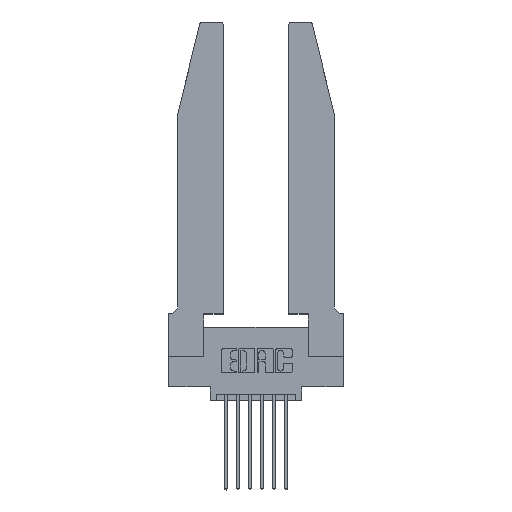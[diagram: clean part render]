
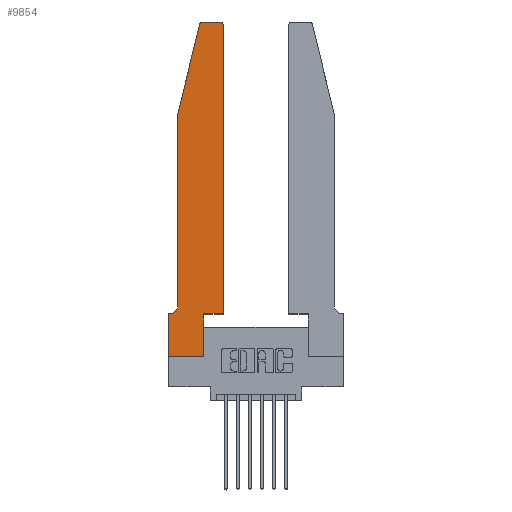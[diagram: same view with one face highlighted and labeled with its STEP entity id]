
A CAD part, top view. The second image highlights one B-rep face of the part: STEP entity #9854.
In plain terms, the highlighted planar face has unit normal (0, 0, 1).
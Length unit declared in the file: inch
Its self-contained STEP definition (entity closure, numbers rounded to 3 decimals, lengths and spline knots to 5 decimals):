
#182 = VECTOR ( 'NONE', #11333, 39.37008 ) ;
#217 = DIRECTION ( 'NONE',  ( 0., 0., 1. ) ) ;
#329 = EDGE_CURVE ( 'NONE', #9574, #2179, #9355, .T. ) ;
#673 = VECTOR ( 'NONE', #8299, 39.37008 ) ;
#785 = ORIENTED_EDGE ( 'NONE', *, *, #9472, .T. ) ;
#1002 = LINE ( 'NONE', #8982, #1178 ) ;
#1145 = EDGE_CURVE ( 'NONE', #2179, #4719, #1292, .T. ) ;
#1178 = VECTOR ( 'NONE', #5602, 39.37008 ) ;
#1292 = LINE ( 'NONE', #14469, #14394 ) ;
#1316 = DIRECTION ( 'NONE',  ( 1., 0., 0. ) ) ;
#1964 = ORIENTED_EDGE ( 'NONE', *, *, #12261, .T. ) ;
#2009 = CARTESIAN_POINT ( 'NONE',  ( 0.25487, 2.72718, 0.37 ) ) ;
#2179 = VERTEX_POINT ( 'NONE', #2859 ) ;
#2706 = CARTESIAN_POINT ( 'NONE',  ( 0.2865, 0., 0.37 ) ) ;
#2859 = CARTESIAN_POINT ( 'NONE',  ( 0.0055, 0.35, 0.37 ) ) ;
#3103 = LINE ( 'NONE', #12303, #9683 ) ;
#3214 = CARTESIAN_POINT ( 'NONE',  ( 0.2865, 0.35, 0.37 ) ) ;
#3313 = PLANE ( 'NONE',  #5761 ) ;
#3316 = VERTEX_POINT ( 'NONE', #2706 ) ;
#3802 = CIRCLE ( 'NONE', #13744, 0.03 ) ;
#3925 = CARTESIAN_POINT ( 'NONE',  ( 0.4505, 0.35, 0.37 ) ) ;
#3987 = LINE ( 'NONE', #7133, #673 ) ;
#4119 = CARTESIAN_POINT ( 'NONE',  ( 0., 0., 0.37 ) ) ;
#4132 = FACE_OUTER_BOUND ( 'NONE', #8071, .T. ) ;
#4164 = VECTOR ( 'NONE', #7392, 39.37008 ) ;
#4212 = VERTEX_POINT ( 'NONE', #10690 ) ;
#4330 = ORIENTED_EDGE ( 'NONE', *, *, #10019, .T. ) ;
#4646 = VECTOR ( 'NONE', #11524, 39.37008 ) ;
#4649 = DIRECTION ( 'NONE',  ( -0.239, -0.971, 0. ) ) ;
#4719 = VERTEX_POINT ( 'NONE', #6005 ) ;
#4817 = VERTEX_POINT ( 'NONE', #4119 ) ;
#4819 = LINE ( 'NONE', #10349, #6881 ) ;
#5023 = EDGE_CURVE ( 'NONE', #11621, #13832, #3103, .T. ) ;
#5448 = EDGE_CURVE ( 'NONE', #3316, #9786, #7367, .T. ) ;
#5484 = CARTESIAN_POINT ( 'NONE',  ( 0.0755, 0.42, 0.37 ) ) ;
#5602 = DIRECTION ( 'NONE',  ( -1., 0., 0. ) ) ;
#5709 = DIRECTION ( 'NONE',  ( 0., 0., -1. ) ) ;
#5761 = AXIS2_PLACEMENT_3D ( 'NONE', #13347, #9991, #11146 ) ;
#5821 = ORIENTED_EDGE ( 'NONE', *, *, #11363, .T. ) ;
#6005 = CARTESIAN_POINT ( 'NONE',  ( 0., 0.35, 0.37 ) ) ;
#6082 = ORIENTED_EDGE ( 'NONE', *, *, #7793, .T. ) ;
#6100 = ORIENTED_EDGE ( 'NONE', *, *, #5448, .T. ) ;
#6203 = ORIENTED_EDGE ( 'NONE', *, *, #1145, .T. ) ;
#6380 = AXIS2_PLACEMENT_3D ( 'NONE', #10521, #10358, #11460 ) ;
#6488 = CARTESIAN_POINT ( 'NONE',  ( 0., 0., 0.37 ) ) ;
#6531 = VECTOR ( 'NONE', #1316, 39.37008 ) ;
#6545 = VERTEX_POINT ( 'NONE', #3925 ) ;
#6563 = DIRECTION ( 'NONE',  ( -1., 0., 0. ) ) ;
#6828 = CARTESIAN_POINT ( 'NONE',  ( 0.4505, 0.35, 0.37 ) ) ;
#6881 = VECTOR ( 'NONE', #9256, 39.37008 ) ;
#7117 = CARTESIAN_POINT ( 'NONE',  ( 0.4505, 2.72, 0.37 ) ) ;
#7123 = CARTESIAN_POINT ( 'NONE',  ( 0.2865, 0.35, 0.37 ) ) ;
#7133 = CARTESIAN_POINT ( 'NONE',  ( 0.0755, 2., 0.37 ) ) ;
#7349 = VERTEX_POINT ( 'NONE', #7117 ) ;
#7367 = LINE ( 'NONE', #7123, #4646 ) ;
#7392 = DIRECTION ( 'NONE',  ( 1., 0., 0. ) ) ;
#7728 = ORIENTED_EDGE ( 'NONE', *, *, #14034, .T. ) ;
#7793 = EDGE_CURVE ( 'NONE', #4719, #4817, #9917, .T. ) ;
#7914 = CARTESIAN_POINT ( 'NONE',  ( 0.0055, 0.42, 0.37 ) ) ;
#8071 = EDGE_LOOP ( 'NONE', ( #4330, #5821, #10670, #785, #14130, #6203, #6082, #1964, #6100, #9802, #7728, #11870 ) ) ;
#8299 = DIRECTION ( 'NONE',  ( 0., -1., 0. ) ) ;
#8711 = CARTESIAN_POINT ( 'NONE',  ( 0.0755, 2., 0.37 ) ) ;
#8782 = LINE ( 'NONE', #6828, #6531 ) ;
#8850 = CARTESIAN_POINT ( 'NONE',  ( 0.4205, 2.75, 0.37 ) ) ;
#8969 = EDGE_CURVE ( 'NONE', #7349, #14259, #10765, .T. ) ;
#8982 = CARTESIAN_POINT ( 'NONE',  ( 0.2605, 2.75, 0.37 ) ) ;
#9036 = CARTESIAN_POINT ( 'NONE',  ( 0., 0., 0.37 ) ) ;
#9256 = DIRECTION ( 'NONE',  ( 0., 1., 0. ) ) ;
#9355 = CIRCLE ( 'NONE', #9474, 0.07 ) ;
#9472 = EDGE_CURVE ( 'NONE', #13832, #9574, #3987, .T. ) ;
#9474 = AXIS2_PLACEMENT_3D ( 'NONE', #7914, #5709, #12305 ) ;
#9574 = VERTEX_POINT ( 'NONE', #5484 ) ;
#9683 = VECTOR ( 'NONE', #4649, 39.37008 ) ;
#9786 = VERTEX_POINT ( 'NONE', #3214 ) ;
#9802 = ORIENTED_EDGE ( 'NONE', *, *, #10218, .T. ) ;
#9854 = ADVANCED_FACE ( 'NONE', ( #4132 ), #3313, .T. ) ;
#9917 = LINE ( 'NONE', #9036, #182 ) ;
#9991 = DIRECTION ( 'NONE',  ( 0., 0., 1. ) ) ;
#10019 = EDGE_CURVE ( 'NONE', #14259, #4212, #1002, .T. ) ;
#10218 = EDGE_CURVE ( 'NONE', #9786, #6545, #8782, .T. ) ;
#10266 = LINE ( 'NONE', #6488, #4164 ) ;
#10349 = CARTESIAN_POINT ( 'NONE',  ( 0.4505, 0.35, 0.37 ) ) ;
#10358 = DIRECTION ( 'NONE',  ( 0., 0., 1. ) ) ;
#10521 = CARTESIAN_POINT ( 'NONE',  ( 0.4205, 2.72, 0.37 ) ) ;
#10670 = ORIENTED_EDGE ( 'NONE', *, *, #5023, .T. ) ;
#10690 = CARTESIAN_POINT ( 'NONE',  ( 0.284, 2.75, 0.37 ) ) ;
#10765 = CIRCLE ( 'NONE', #6380, 0.03 ) ;
#11146 = DIRECTION ( 'NONE',  ( 1., 0., 0. ) ) ;
#11330 = CARTESIAN_POINT ( 'NONE',  ( 0.284, 2.72, 0.37 ) ) ;
#11333 = DIRECTION ( 'NONE',  ( 0., -1., 0. ) ) ;
#11363 = EDGE_CURVE ( 'NONE', #4212, #11621, #3802, .T. ) ;
#11377 = DIRECTION ( 'NONE',  ( 1., 0., 0. ) ) ;
#11460 = DIRECTION ( 'NONE',  ( 1., 0., 0. ) ) ;
#11524 = DIRECTION ( 'NONE',  ( 0., 1., 0. ) ) ;
#11621 = VERTEX_POINT ( 'NONE', #2009 ) ;
#11870 = ORIENTED_EDGE ( 'NONE', *, *, #8969, .T. ) ;
#12261 = EDGE_CURVE ( 'NONE', #4817, #3316, #10266, .T. ) ;
#12303 = CARTESIAN_POINT ( 'NONE',  ( 0.0755, 2., 0.37 ) ) ;
#12305 = DIRECTION ( 'NONE',  ( -1., 0., 0. ) ) ;
#13347 = CARTESIAN_POINT ( 'NONE',  ( 0., 0.35, 0.37 ) ) ;
#13744 = AXIS2_PLACEMENT_3D ( 'NONE', #11330, #217, #11377 ) ;
#13832 = VERTEX_POINT ( 'NONE', #8711 ) ;
#14034 = EDGE_CURVE ( 'NONE', #6545, #7349, #4819, .T. ) ;
#14130 = ORIENTED_EDGE ( 'NONE', *, *, #329, .T. ) ;
#14259 = VERTEX_POINT ( 'NONE', #8850 ) ;
#14394 = VECTOR ( 'NONE', #6563, 39.37008 ) ;
#14469 = CARTESIAN_POINT ( 'NONE',  ( 0.0755, 0.35, 0.37 ) ) ;
